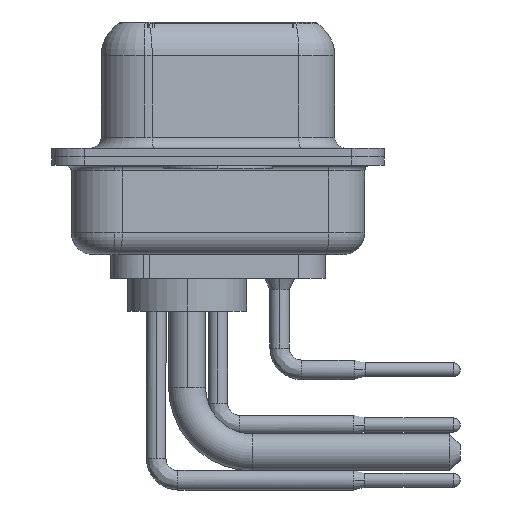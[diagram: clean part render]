
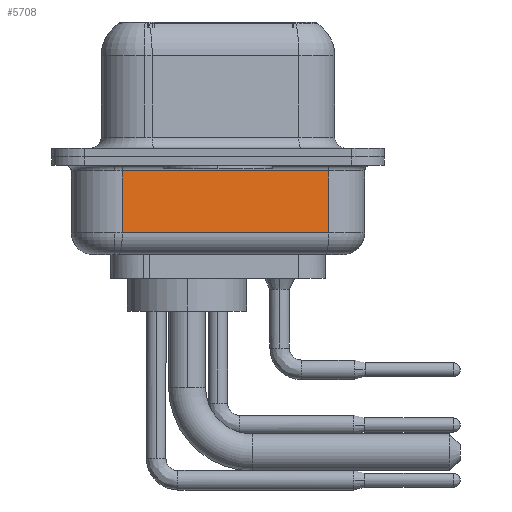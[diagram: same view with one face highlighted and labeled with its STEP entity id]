
A CAD part, left-side view. The second image highlights one B-rep face of the part: STEP entity #5708.
In plain terms, the highlighted planar face has unit normal (-0.985, -0.174, 0).
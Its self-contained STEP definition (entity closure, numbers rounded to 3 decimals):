
#1279 = LINE ( 'NONE', #13957, #2235 ) ;
#1550 = LINE ( 'NONE', #27051, #22884 ) ;
#1665 = VECTOR ( 'NONE', #13275, 1000. ) ;
#2131 = VECTOR ( 'NONE', #23002, 1000. ) ;
#2235 = VECTOR ( 'NONE', #5056, 1000. ) ;
#2686 = VERTEX_POINT ( 'NONE', #23240 ) ;
#4027 = VERTEX_POINT ( 'NONE', #15314 ) ;
#5056 = DIRECTION ( 'NONE',  ( 0., 0., 1. ) ) ;
#5204 = EDGE_CURVE ( 'NONE', #23356, #4027, #17005, .T. ) ;
#5708 = ADVANCED_FACE ( 'NONE', ( #8211 ), #27427, .F. ) ;
#5810 = ORIENTED_EDGE ( 'NONE', *, *, #24949, .T. ) ;
#6401 = DIRECTION ( 'NONE',  ( 0.985, 0.174, 0. ) ) ;
#6760 = EDGE_CURVE ( 'NONE', #13644, #2686, #1279, .T. ) ;
#8211 = FACE_OUTER_BOUND ( 'NONE', #15003, .T. ) ;
#8961 = LINE ( 'NONE', #17450, #1665 ) ;
#10183 = ORIENTED_EDGE ( 'NONE', *, *, #16151, .T. ) ;
#10571 = DIRECTION ( 'NONE',  ( -0.174, 0.985, 0. ) ) ;
#10779 = CARTESIAN_POINT ( 'NONE',  ( 4.605, -5.097, -3.5 ) ) ;
#13275 = DIRECTION ( 'NONE',  ( 0.174, -0.985, 0. ) ) ;
#13644 = VERTEX_POINT ( 'NONE', #18492 ) ;
#13957 = CARTESIAN_POINT ( 'NONE',  ( 2.93, 4.403, -4.5 ) ) ;
#14762 = CARTESIAN_POINT ( 'NONE',  ( 2.93, 4.403, -4.5 ) ) ;
#15003 = EDGE_LOOP ( 'NONE', ( #23355, #10183, #24522, #5810 ) ) ;
#15314 = CARTESIAN_POINT ( 'NONE',  ( 4.605, -5.097, -0.65 ) ) ;
#16151 = EDGE_CURVE ( 'NONE', #13644, #23356, #8961, .T. ) ;
#17005 = LINE ( 'NONE', #18828, #2131 ) ;
#17450 = CARTESIAN_POINT ( 'NONE',  ( 2.93, 4.403, -3.5 ) ) ;
#18492 = CARTESIAN_POINT ( 'NONE',  ( 2.93, 4.403, -3.5 ) ) ;
#18828 = CARTESIAN_POINT ( 'NONE',  ( 4.605, -5.097, -4.5 ) ) ;
#22884 = VECTOR ( 'NONE', #25233, 1000. ) ;
#23002 = DIRECTION ( 'NONE',  ( 0., 0., 1. ) ) ;
#23240 = CARTESIAN_POINT ( 'NONE',  ( 2.93, 4.403, -0.65 ) ) ;
#23355 = ORIENTED_EDGE ( 'NONE', *, *, #6760, .F. ) ;
#23356 = VERTEX_POINT ( 'NONE', #10779 ) ;
#23519 = AXIS2_PLACEMENT_3D ( 'NONE', #14762, #6401, #10571 ) ;
#24522 = ORIENTED_EDGE ( 'NONE', *, *, #5204, .T. ) ;
#24949 = EDGE_CURVE ( 'NONE', #4027, #2686, #1550, .T. ) ;
#25233 = DIRECTION ( 'NONE',  ( -0.174, 0.985, 0. ) ) ;
#27051 = CARTESIAN_POINT ( 'NONE',  ( 2.93, 4.403, -0.65 ) ) ;
#27427 = PLANE ( 'NONE',  #23519 ) ;
